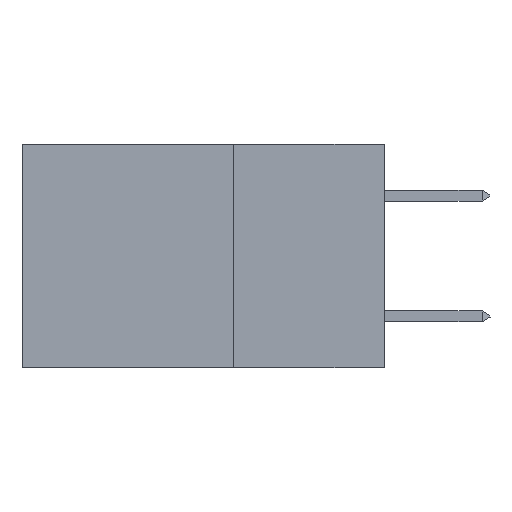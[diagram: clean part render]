
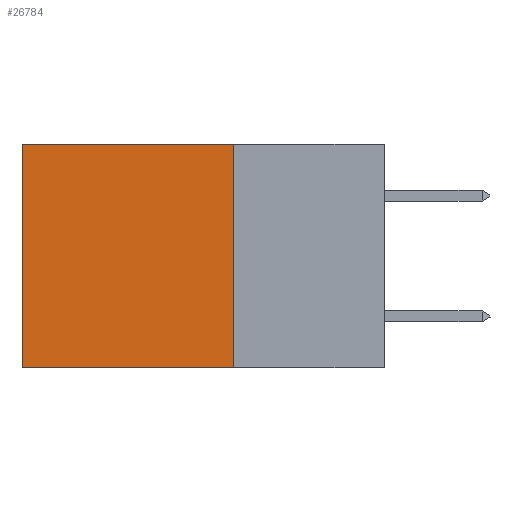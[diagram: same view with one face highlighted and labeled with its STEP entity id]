
A CAD part, left-side view. The second image highlights one B-rep face of the part: STEP entity #26784.
In plain terms, the highlighted planar face has unit normal (-1, 0, 0).
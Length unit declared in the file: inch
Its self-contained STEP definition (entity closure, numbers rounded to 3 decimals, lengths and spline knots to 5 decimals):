
#213 = EDGE_LOOP ( 'NONE', ( #9741, #18547, #20107, #7592 ) ) ;
#4549 = DIRECTION ( 'NONE',  ( 0., 0., -1. ) ) ;
#4727 = AXIS2_PLACEMENT_3D ( 'NONE', #16836, #8299, #27273 ) ;
#4954 = EDGE_CURVE ( 'NONE', #8371, #11896, #9031, .T. ) ;
#5536 = DIRECTION ( 'NONE',  ( 0., 1., 0. ) ) ;
#5777 = CARTESIAN_POINT ( 'NONE',  ( 0.2875, 0.6, 0. ) ) ;
#6338 = CARTESIAN_POINT ( 'NONE',  ( 0.2875, 0.6, 0. ) ) ;
#6940 = CARTESIAN_POINT ( 'NONE',  ( 0.2875, 0.25, 0. ) ) ;
#7592 = ORIENTED_EDGE ( 'NONE', *, *, #4954, .T. ) ;
#8299 = DIRECTION ( 'NONE',  ( 1., 0., 0. ) ) ;
#8371 = VERTEX_POINT ( 'NONE', #9097 ) ;
#9031 = LINE ( 'NONE', #6940, #10705 ) ;
#9097 = CARTESIAN_POINT ( 'NONE',  ( 0.2875, 0.25, 0. ) ) ;
#9741 = ORIENTED_EDGE ( 'NONE', *, *, #19202, .T. ) ;
#10705 = VECTOR ( 'NONE', #5536, 39.37008 ) ;
#10955 = DIRECTION ( 'NONE',  ( 0., 1., 0. ) ) ;
#11896 = VERTEX_POINT ( 'NONE', #5777 ) ;
#12033 = LINE ( 'NONE', #23968, #25418 ) ;
#13529 = CARTESIAN_POINT ( 'NONE',  ( 0.2875, 0.25, -0.37 ) ) ;
#13563 = VECTOR ( 'NONE', #4549, 39.37008 ) ;
#15661 = CARTESIAN_POINT ( 'NONE',  ( 0.2875, 0.6, -0.37 ) ) ;
#16836 = CARTESIAN_POINT ( 'NONE',  ( 0.2875, 0.25, 0. ) ) ;
#16919 = LINE ( 'NONE', #23672, #13563 ) ;
#18082 = VERTEX_POINT ( 'NONE', #13529 ) ;
#18547 = ORIENTED_EDGE ( 'NONE', *, *, #22237, .F. ) ;
#18594 = FACE_OUTER_BOUND ( 'NONE', #213, .T. ) ;
#19202 = EDGE_CURVE ( 'NONE', #11896, #27674, #23899, .T. ) ;
#19357 = DIRECTION ( 'NONE',  ( 0., 0., -1. ) ) ;
#20107 = ORIENTED_EDGE ( 'NONE', *, *, #25238, .F. ) ;
#21258 = VECTOR ( 'NONE', #19357, 39.37008 ) ;
#22237 = EDGE_CURVE ( 'NONE', #18082, #27674, #12033, .T. ) ;
#23672 = CARTESIAN_POINT ( 'NONE',  ( 0.2875, 0.25, 0. ) ) ;
#23899 = LINE ( 'NONE', #6338, #21258 ) ;
#23968 = CARTESIAN_POINT ( 'NONE',  ( 0.2875, 0.25, -0.37 ) ) ;
#25238 = EDGE_CURVE ( 'NONE', #8371, #18082, #16919, .T. ) ;
#25349 = PLANE ( 'NONE',  #4727 ) ;
#25418 = VECTOR ( 'NONE', #10955, 39.37008 ) ;
#26784 = ADVANCED_FACE ( 'NONE', ( #18594 ), #25349, .F. ) ;
#27273 = DIRECTION ( 'NONE',  ( 0., 0., -1. ) ) ;
#27674 = VERTEX_POINT ( 'NONE', #15661 ) ;
